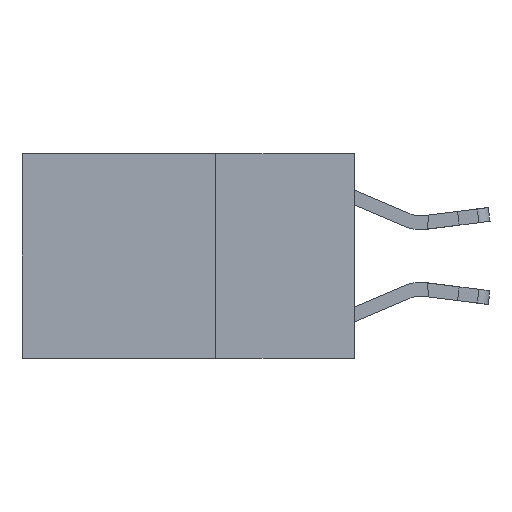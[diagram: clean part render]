
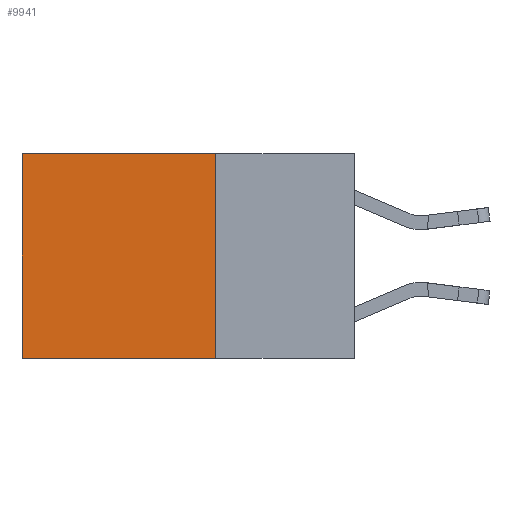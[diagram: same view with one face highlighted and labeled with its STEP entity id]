
A CAD part, left-side view. The second image highlights one B-rep face of the part: STEP entity #9941.
In plain terms, the highlighted planar face has unit normal (-1, 0, 0).
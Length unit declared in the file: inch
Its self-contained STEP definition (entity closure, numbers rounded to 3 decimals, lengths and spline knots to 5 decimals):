
#179 = EDGE_CURVE ( 'NONE', #10867, #6968, #3338, .T. ) ;
#439 = EDGE_LOOP ( 'NONE', ( #8505, #10608, #8453, #7655 ) ) ;
#539 = DIRECTION ( 'NONE',  ( 0., 0., -1. ) ) ;
#857 = VECTOR ( 'NONE', #12416, 39.37008 ) ;
#1441 = DIRECTION ( 'NONE',  ( 1., 0., 0. ) ) ;
#2919 = CARTESIAN_POINT ( 'NONE',  ( 0.2625, 0.25, 0. ) ) ;
#3265 = VERTEX_POINT ( 'NONE', #7188 ) ;
#3338 = LINE ( 'NONE', #7224, #4464 ) ;
#3430 = CARTESIAN_POINT ( 'NONE',  ( 0.2625, 0.25, 0. ) ) ;
#3993 = DIRECTION ( 'NONE',  ( 0., 0., -1. ) ) ;
#4144 = CARTESIAN_POINT ( 'NONE',  ( 0.2625, 0.6, -0.37 ) ) ;
#4325 = FACE_OUTER_BOUND ( 'NONE', #439, .T. ) ;
#4464 = VECTOR ( 'NONE', #11137, 39.37008 ) ;
#4735 = CARTESIAN_POINT ( 'NONE',  ( 0.2625, 0.25, 0. ) ) ;
#5777 = VECTOR ( 'NONE', #9313, 39.37008 ) ;
#6394 = LINE ( 'NONE', #10279, #5777 ) ;
#6572 = CARTESIAN_POINT ( 'NONE',  ( 0.2625, 0.6, 0. ) ) ;
#6968 = VERTEX_POINT ( 'NONE', #4144 ) ;
#7188 = CARTESIAN_POINT ( 'NONE',  ( 0.2625, 0.25, -0.37 ) ) ;
#7224 = CARTESIAN_POINT ( 'NONE',  ( 0.2625, 0.6, 0. ) ) ;
#7595 = LINE ( 'NONE', #4735, #857 ) ;
#7655 = ORIENTED_EDGE ( 'NONE', *, *, #7848, .T. ) ;
#7746 = LINE ( 'NONE', #2919, #10600 ) ;
#7848 = EDGE_CURVE ( 'NONE', #10593, #10867, #7595, .T. ) ;
#7960 = CARTESIAN_POINT ( 'NONE',  ( 0.2625, 0.25, 0. ) ) ;
#8161 = EDGE_CURVE ( 'NONE', #3265, #6968, #6394, .T. ) ;
#8453 = ORIENTED_EDGE ( 'NONE', *, *, #9317, .F. ) ;
#8505 = ORIENTED_EDGE ( 'NONE', *, *, #179, .T. ) ;
#9313 = DIRECTION ( 'NONE',  ( 0., 1., 0. ) ) ;
#9317 = EDGE_CURVE ( 'NONE', #10593, #3265, #7746, .T. ) ;
#9941 = ADVANCED_FACE ( 'NONE', ( #4325 ), #12191, .F. ) ;
#10279 = CARTESIAN_POINT ( 'NONE',  ( 0.2625, 0.25, -0.37 ) ) ;
#10593 = VERTEX_POINT ( 'NONE', #7960 ) ;
#10600 = VECTOR ( 'NONE', #3993, 39.37008 ) ;
#10608 = ORIENTED_EDGE ( 'NONE', *, *, #8161, .F. ) ;
#10867 = VERTEX_POINT ( 'NONE', #6572 ) ;
#11137 = DIRECTION ( 'NONE',  ( 0., 0., -1. ) ) ;
#11654 = AXIS2_PLACEMENT_3D ( 'NONE', #3430, #1441, #539 ) ;
#12191 = PLANE ( 'NONE',  #11654 ) ;
#12416 = DIRECTION ( 'NONE',  ( 0., 1., 0. ) ) ;
